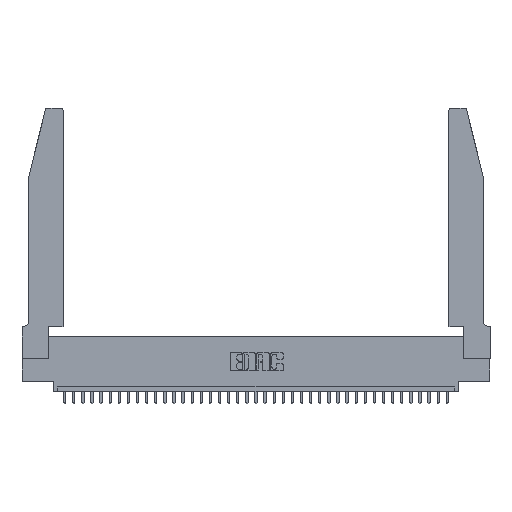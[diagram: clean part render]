
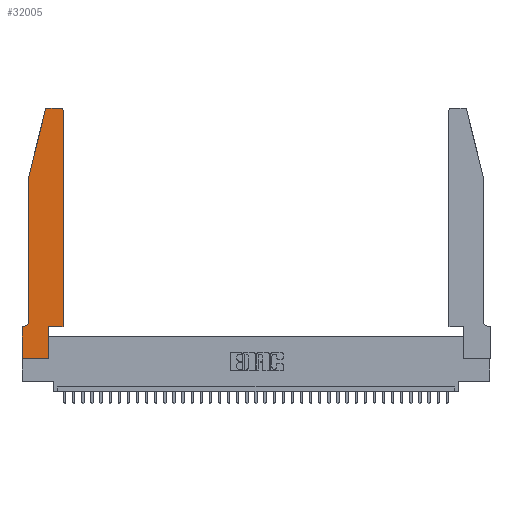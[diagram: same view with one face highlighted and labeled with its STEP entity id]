
A CAD part, top view. The second image highlights one B-rep face of the part: STEP entity #32005.
In plain terms, the highlighted planar face has unit normal (0, 0, 1).
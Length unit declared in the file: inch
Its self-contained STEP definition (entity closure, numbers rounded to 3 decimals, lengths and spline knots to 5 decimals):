
#984 = CARTESIAN_POINT ( 'NONE',  ( 0.0755, 0.35, 0.37 ) ) ;
#995 = DIRECTION ( 'NONE',  ( 0., -1., 0. ) ) ;
#1158 = PLANE ( 'NONE',  #21943 ) ;
#3015 = CARTESIAN_POINT ( 'NONE',  ( 0.0055, 0.35, 0.37 ) ) ;
#3114 = LINE ( 'NONE', #10481, #13481 ) ;
#3928 = LINE ( 'NONE', #33389, #4872 ) ;
#4059 = CARTESIAN_POINT ( 'NONE',  ( 0., 0.35, 0.37 ) ) ;
#4566 = VERTEX_POINT ( 'NONE', #10766 ) ;
#4872 = VECTOR ( 'NONE', #27593, 39.37008 ) ;
#5761 = ORIENTED_EDGE ( 'NONE', *, *, #32253, .T. ) ;
#5827 = CIRCLE ( 'NONE', #7244, 0.03 ) ;
#6038 = CARTESIAN_POINT ( 'NONE',  ( 0.4505, 0.35, 0.37 ) ) ;
#6552 = EDGE_CURVE ( 'NONE', #9514, #20393, #5827, .T. ) ;
#6561 = CARTESIAN_POINT ( 'NONE',  ( 0.284, 2.72, 0.37 ) ) ;
#6713 = VERTEX_POINT ( 'NONE', #29747 ) ;
#6788 = ORIENTED_EDGE ( 'NONE', *, *, #35936, .T. ) ;
#6972 = ORIENTED_EDGE ( 'NONE', *, *, #6552, .T. ) ;
#7149 = VERTEX_POINT ( 'NONE', #14109 ) ;
#7244 = AXIS2_PLACEMENT_3D ( 'NONE', #6561, #13231, #7562 ) ;
#7562 = DIRECTION ( 'NONE',  ( 1., 0., 0. ) ) ;
#7655 = LINE ( 'NONE', #984, #16243 ) ;
#7753 = ORIENTED_EDGE ( 'NONE', *, *, #30981, .T. ) ;
#8589 = CARTESIAN_POINT ( 'NONE',  ( 0.25487, 2.72718, 0.37 ) ) ;
#9004 = EDGE_CURVE ( 'NONE', #9738, #7149, #35265, .T. ) ;
#9513 = ORIENTED_EDGE ( 'NONE', *, *, #22526, .T. ) ;
#9514 = VERTEX_POINT ( 'NONE', #19049 ) ;
#9688 = DIRECTION ( 'NONE',  ( 0., 0., 1. ) ) ;
#9738 = VERTEX_POINT ( 'NONE', #32221 ) ;
#9864 = CARTESIAN_POINT ( 'NONE',  ( 0.0755, 2., 0.37 ) ) ;
#10030 = VERTEX_POINT ( 'NONE', #30730 ) ;
#10481 = CARTESIAN_POINT ( 'NONE',  ( 0.4505, 0.35, 0.37 ) ) ;
#10663 = CIRCLE ( 'NONE', #26433, 0.03 ) ;
#10766 = CARTESIAN_POINT ( 'NONE',  ( 0.2865, 0.35, 0.37 ) ) ;
#11891 = VERTEX_POINT ( 'NONE', #13035 ) ;
#12215 = EDGE_CURVE ( 'NONE', #6713, #10030, #3114, .T. ) ;
#13035 = CARTESIAN_POINT ( 'NONE',  ( 0.4205, 2.75, 0.37 ) ) ;
#13231 = DIRECTION ( 'NONE',  ( 0., 0., 1. ) ) ;
#13337 = VERTEX_POINT ( 'NONE', #36098 ) ;
#13473 = LINE ( 'NONE', #27056, #27294 ) ;
#13481 = VECTOR ( 'NONE', #34000, 39.37008 ) ;
#14109 = CARTESIAN_POINT ( 'NONE',  ( 0., 0., 0.37 ) ) ;
#14980 = LINE ( 'NONE', #24183, #21697 ) ;
#16243 = VECTOR ( 'NONE', #21089, 39.37008 ) ;
#16385 = VERTEX_POINT ( 'NONE', #9864 ) ;
#17130 = LINE ( 'NONE', #6038, #35013 ) ;
#17138 = CARTESIAN_POINT ( 'NONE',  ( 0., 0., 0.37 ) ) ;
#17827 = CARTESIAN_POINT ( 'NONE',  ( 0.2865, 0., 0.37 ) ) ;
#18628 = DIRECTION ( 'NONE',  ( -1., 0., 0. ) ) ;
#18708 = DIRECTION ( 'NONE',  ( 0., 1., 0. ) ) ;
#19049 = CARTESIAN_POINT ( 'NONE',  ( 0.284, 2.75, 0.37 ) ) ;
#19161 = ORIENTED_EDGE ( 'NONE', *, *, #35997, .T. ) ;
#19172 = VECTOR ( 'NONE', #995, 39.37008 ) ;
#19381 = DIRECTION ( 'NONE',  ( 1., 0., 0. ) ) ;
#19503 = CARTESIAN_POINT ( 'NONE',  ( 0.2605, 2.75, 0.37 ) ) ;
#19820 = AXIS2_PLACEMENT_3D ( 'NONE', #27467, #21484, #18628 ) ;
#20393 = VERTEX_POINT ( 'NONE', #8589 ) ;
#20816 = EDGE_CURVE ( 'NONE', #16385, #13337, #3928, .T. ) ;
#20844 = ORIENTED_EDGE ( 'NONE', *, *, #22611, .T. ) ;
#20999 = DIRECTION ( 'NONE',  ( 1., 0., 0. ) ) ;
#21089 = DIRECTION ( 'NONE',  ( -1., 0., 0. ) ) ;
#21484 = DIRECTION ( 'NONE',  ( 0., 0., -1. ) ) ;
#21574 = DIRECTION ( 'NONE',  ( -0.239, -0.971, 0. ) ) ;
#21697 = VECTOR ( 'NONE', #18708, 39.37008 ) ;
#21943 = AXIS2_PLACEMENT_3D ( 'NONE', #4059, #24114, #26965 ) ;
#21980 = LINE ( 'NONE', #25092, #31845 ) ;
#22371 = DIRECTION ( 'NONE',  ( -1., 0., 0. ) ) ;
#22526 = EDGE_CURVE ( 'NONE', #10030, #11891, #10663, .T. ) ;
#22611 = EDGE_CURVE ( 'NONE', #13337, #30689, #36593, .T. ) ;
#22808 = ORIENTED_EDGE ( 'NONE', *, *, #27272, .T. ) ;
#24061 = VERTEX_POINT ( 'NONE', #17827 ) ;
#24114 = DIRECTION ( 'NONE',  ( 0., 0., 1. ) ) ;
#24160 = ORIENTED_EDGE ( 'NONE', *, *, #27642, .T. ) ;
#24183 = CARTESIAN_POINT ( 'NONE',  ( 0.2865, 0.35, 0.37 ) ) ;
#25092 = CARTESIAN_POINT ( 'NONE',  ( 0., 0., 0.37 ) ) ;
#26433 = AXIS2_PLACEMENT_3D ( 'NONE', #26825, #9688, #20999 ) ;
#26537 = FACE_OUTER_BOUND ( 'NONE', #36137, .T. ) ;
#26825 = CARTESIAN_POINT ( 'NONE',  ( 0.4205, 2.72, 0.37 ) ) ;
#26965 = DIRECTION ( 'NONE',  ( 1., 0., 0. ) ) ;
#27056 = CARTESIAN_POINT ( 'NONE',  ( 0.0755, 2., 0.37 ) ) ;
#27272 = EDGE_CURVE ( 'NONE', #7149, #24061, #21980, .T. ) ;
#27294 = VECTOR ( 'NONE', #21574, 39.37008 ) ;
#27467 = CARTESIAN_POINT ( 'NONE',  ( 0.0055, 0.42, 0.37 ) ) ;
#27593 = DIRECTION ( 'NONE',  ( 0., -1., 0. ) ) ;
#27642 = EDGE_CURVE ( 'NONE', #20393, #16385, #13473, .T. ) ;
#28779 = VECTOR ( 'NONE', #22371, 39.37008 ) ;
#29747 = CARTESIAN_POINT ( 'NONE',  ( 0.4505, 0.35, 0.37 ) ) ;
#30689 = VERTEX_POINT ( 'NONE', #3015 ) ;
#30730 = CARTESIAN_POINT ( 'NONE',  ( 0.4505, 2.72, 0.37 ) ) ;
#30981 = EDGE_CURVE ( 'NONE', #24061, #4566, #14980, .T. ) ;
#31845 = VECTOR ( 'NONE', #19381, 39.37008 ) ;
#32005 = ADVANCED_FACE ( 'NONE', ( #26537 ), #1158, .T. ) ;
#32221 = CARTESIAN_POINT ( 'NONE',  ( 0., 0.35, 0.37 ) ) ;
#32253 = EDGE_CURVE ( 'NONE', #11891, #9514, #34603, .T. ) ;
#32825 = ORIENTED_EDGE ( 'NONE', *, *, #12215, .T. ) ;
#33389 = CARTESIAN_POINT ( 'NONE',  ( 0.0755, 2., 0.37 ) ) ;
#34000 = DIRECTION ( 'NONE',  ( 0., 1., 0. ) ) ;
#34559 = ORIENTED_EDGE ( 'NONE', *, *, #20816, .T. ) ;
#34603 = LINE ( 'NONE', #19503, #28779 ) ;
#35013 = VECTOR ( 'NONE', #35346, 39.37008 ) ;
#35265 = LINE ( 'NONE', #17138, #19172 ) ;
#35346 = DIRECTION ( 'NONE',  ( 1., 0., 0. ) ) ;
#35868 = ORIENTED_EDGE ( 'NONE', *, *, #9004, .T. ) ;
#35936 = EDGE_CURVE ( 'NONE', #4566, #6713, #17130, .T. ) ;
#35997 = EDGE_CURVE ( 'NONE', #30689, #9738, #7655, .T. ) ;
#36098 = CARTESIAN_POINT ( 'NONE',  ( 0.0755, 0.42, 0.37 ) ) ;
#36137 = EDGE_LOOP ( 'NONE', ( #5761, #6972, #24160, #34559, #20844, #19161, #35868, #22808, #7753, #6788, #32825, #9513 ) ) ;
#36593 = CIRCLE ( 'NONE', #19820, 0.07 ) ;
